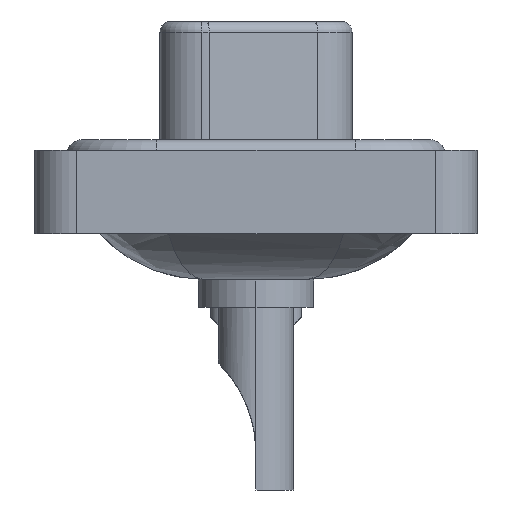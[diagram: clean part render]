
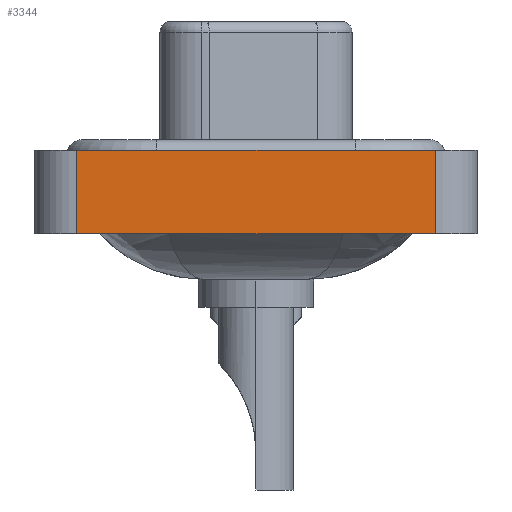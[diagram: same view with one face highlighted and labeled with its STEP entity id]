
A CAD part, left-side view. The second image highlights one B-rep face of the part: STEP entity #3344.
In plain terms, the highlighted planar face has unit normal (-1, 0, 0).
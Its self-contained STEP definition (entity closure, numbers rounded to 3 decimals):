
#1200 = VERTEX_POINT ( 'NONE', #15957 ) ;
#1440 = EDGE_CURVE ( 'NONE', #6693, #15264, #6300, .T. ) ;
#1602 = ORIENTED_EDGE ( 'NONE', *, *, #14795, .F. ) ;
#1774 = DIRECTION ( 'NONE',  ( -1., 0., 0. ) ) ;
#3150 = DIRECTION ( 'NONE',  ( 0., 0., 1. ) ) ;
#3258 = CARTESIAN_POINT ( 'NONE',  ( -7.35, -8.55, -3.6 ) ) ;
#3344 = ADVANCED_FACE ( 'NONE', ( #8958 ), #17150, .T. ) ;
#3965 = EDGE_CURVE ( 'NONE', #1200, #6693, #14425, .T. ) ;
#3978 = CARTESIAN_POINT ( 'NONE',  ( -7.35, -8.55, -3.6 ) ) ;
#3993 = ORIENTED_EDGE ( 'NONE', *, *, #3965, .T. ) ;
#4398 = CARTESIAN_POINT ( 'NONE',  ( -7.35, 8.55, 0.4 ) ) ;
#4794 = LINE ( 'NONE', #11680, #21967 ) ;
#5653 = DIRECTION ( 'NONE',  ( 0., -1., 0. ) ) ;
#6295 = VECTOR ( 'NONE', #10858, 1000. ) ;
#6300 = LINE ( 'NONE', #11914, #21580 ) ;
#6693 = VERTEX_POINT ( 'NONE', #3258 ) ;
#8720 = CARTESIAN_POINT ( 'NONE',  ( -7.35, -8.55, -3.6 ) ) ;
#8958 = FACE_OUTER_BOUND ( 'NONE', #9842, .T. ) ;
#9842 = EDGE_LOOP ( 'NONE', ( #19383, #1602, #12221, #3993 ) ) ;
#10858 = DIRECTION ( 'NONE',  ( 0., -1., 0. ) ) ;
#11680 = CARTESIAN_POINT ( 'NONE',  ( -7.35, 8.55, -3.6 ) ) ;
#11914 = CARTESIAN_POINT ( 'NONE',  ( -7.35, -8.55, -3.6 ) ) ;
#12221 = ORIENTED_EDGE ( 'NONE', *, *, #17719, .F. ) ;
#13179 = VECTOR ( 'NONE', #5653, 1000. ) ;
#14425 = LINE ( 'NONE', #3978, #6295 ) ;
#14795 = EDGE_CURVE ( 'NONE', #16777, #15264, #21381, .T. ) ;
#15264 = VERTEX_POINT ( 'NONE', #17450 ) ;
#15957 = CARTESIAN_POINT ( 'NONE',  ( -7.35, 8.55, -3.6 ) ) ;
#16195 = CARTESIAN_POINT ( 'NONE',  ( -7.35, -8.55, 0.4 ) ) ;
#16777 = VERTEX_POINT ( 'NONE', #4398 ) ;
#17150 = PLANE ( 'NONE',  #17731 ) ;
#17450 = CARTESIAN_POINT ( 'NONE',  ( -7.35, -8.55, 0.4 ) ) ;
#17719 = EDGE_CURVE ( 'NONE', #1200, #16777, #4794, .T. ) ;
#17731 = AXIS2_PLACEMENT_3D ( 'NONE', #8720, #1774, #18939 ) ;
#18491 = DIRECTION ( 'NONE',  ( 0., 0., 1. ) ) ;
#18939 = DIRECTION ( 'NONE',  ( 0., 0., 1. ) ) ;
#19383 = ORIENTED_EDGE ( 'NONE', *, *, #1440, .T. ) ;
#21381 = LINE ( 'NONE', #16195, #13179 ) ;
#21580 = VECTOR ( 'NONE', #3150, 1000. ) ;
#21967 = VECTOR ( 'NONE', #18491, 1000. ) ;
